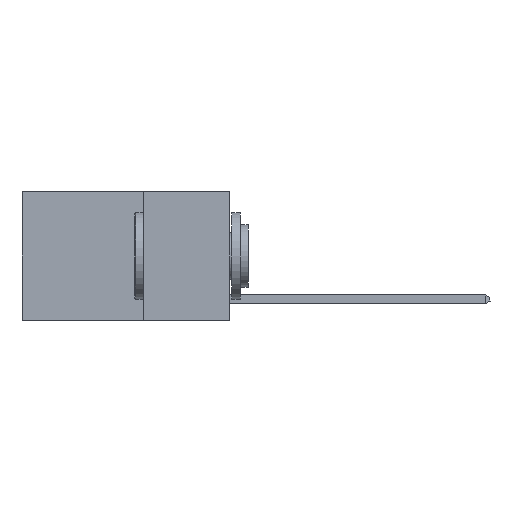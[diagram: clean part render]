
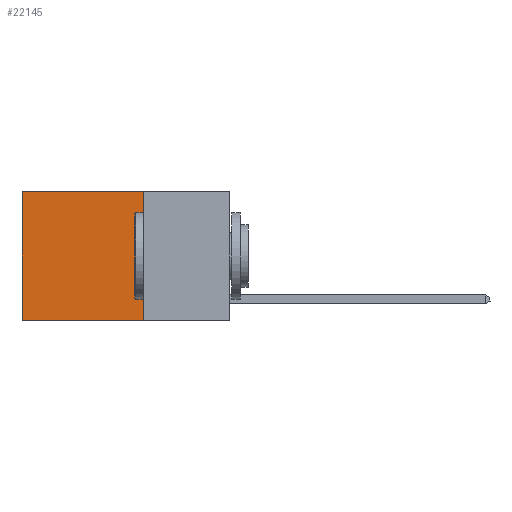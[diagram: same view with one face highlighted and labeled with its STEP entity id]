
A CAD part, left-side view. The second image highlights one B-rep face of the part: STEP entity #22145.
In plain terms, the highlighted planar face has unit normal (-1, 0, 0).
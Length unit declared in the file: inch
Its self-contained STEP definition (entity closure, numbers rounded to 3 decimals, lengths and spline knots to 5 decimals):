
#1599 = CARTESIAN_POINT ( 'NONE',  ( 0.2625, 0.25, -0.37 ) ) ;
#3886 = DIRECTION ( 'NONE',  ( 0., 0., -1. ) ) ;
#4857 = AXIS2_PLACEMENT_3D ( 'NONE', #11203, #9111, #24322 ) ;
#4890 = CARTESIAN_POINT ( 'NONE',  ( 0.2625, 0.6, -0.37 ) ) ;
#6338 = VERTEX_POINT ( 'NONE', #17726 ) ;
#6400 = LINE ( 'NONE', #8159, #23054 ) ;
#6678 = LINE ( 'NONE', #11621, #22641 ) ;
#7349 = DIRECTION ( 'NONE',  ( 0., 1., 0. ) ) ;
#8159 = CARTESIAN_POINT ( 'NONE',  ( 0.2625, 0.25, 0. ) ) ;
#9111 = DIRECTION ( 'NONE',  ( 1., 0., 0. ) ) ;
#9315 = ORIENTED_EDGE ( 'NONE', *, *, #16794, .T. ) ;
#10394 = VERTEX_POINT ( 'NONE', #21660 ) ;
#11086 = VERTEX_POINT ( 'NONE', #21724 ) ;
#11203 = CARTESIAN_POINT ( 'NONE',  ( 0.2625, 0.25, 0. ) ) ;
#11621 = CARTESIAN_POINT ( 'NONE',  ( 0.2625, 0.25, 0. ) ) ;
#12448 = DIRECTION ( 'NONE',  ( 0., 1., 0. ) ) ;
#13046 = CARTESIAN_POINT ( 'NONE',  ( 0.2625, 0.6, 0. ) ) ;
#14126 = EDGE_CURVE ( 'NONE', #10394, #14858, #24847, .T. ) ;
#14235 = ORIENTED_EDGE ( 'NONE', *, *, #24481, .F. ) ;
#14858 = VERTEX_POINT ( 'NONE', #4890 ) ;
#16794 = EDGE_CURVE ( 'NONE', #11086, #10394, #6678, .T. ) ;
#17726 = CARTESIAN_POINT ( 'NONE',  ( 0.2625, 0.25, -0.37 ) ) ;
#18191 = VECTOR ( 'NONE', #12448, 39.37008 ) ;
#19562 = LINE ( 'NONE', #1599, #18191 ) ;
#19932 = PLANE ( 'NONE',  #4857 ) ;
#20295 = ORIENTED_EDGE ( 'NONE', *, *, #26403, .F. ) ;
#20396 = DIRECTION ( 'NONE',  ( 0., 0., -1. ) ) ;
#21345 = FACE_OUTER_BOUND ( 'NONE', #23019, .T. ) ;
#21359 = ORIENTED_EDGE ( 'NONE', *, *, #14126, .T. ) ;
#21660 = CARTESIAN_POINT ( 'NONE',  ( 0.2625, 0.6, 0. ) ) ;
#21724 = CARTESIAN_POINT ( 'NONE',  ( 0.2625, 0.25, 0. ) ) ;
#22145 = ADVANCED_FACE ( 'NONE', ( #21345 ), #19932, .F. ) ;
#22641 = VECTOR ( 'NONE', #7349, 39.37008 ) ;
#23019 = EDGE_LOOP ( 'NONE', ( #21359, #14235, #20295, #9315 ) ) ;
#23054 = VECTOR ( 'NONE', #3886, 39.37008 ) ;
#24182 = VECTOR ( 'NONE', #20396, 39.37008 ) ;
#24322 = DIRECTION ( 'NONE',  ( 0., 0., -1. ) ) ;
#24481 = EDGE_CURVE ( 'NONE', #6338, #14858, #19562, .T. ) ;
#24847 = LINE ( 'NONE', #13046, #24182 ) ;
#26403 = EDGE_CURVE ( 'NONE', #11086, #6338, #6400, .T. ) ;
